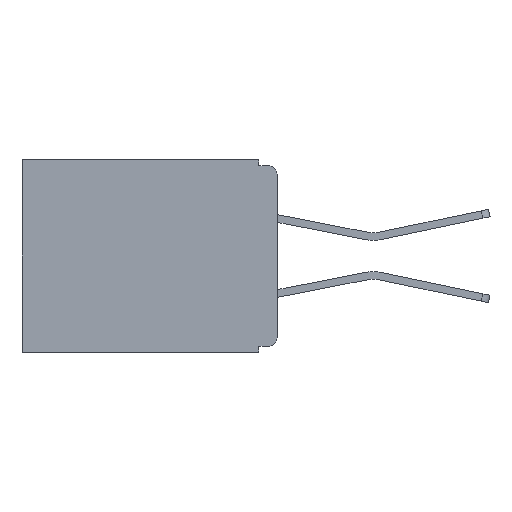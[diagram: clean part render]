
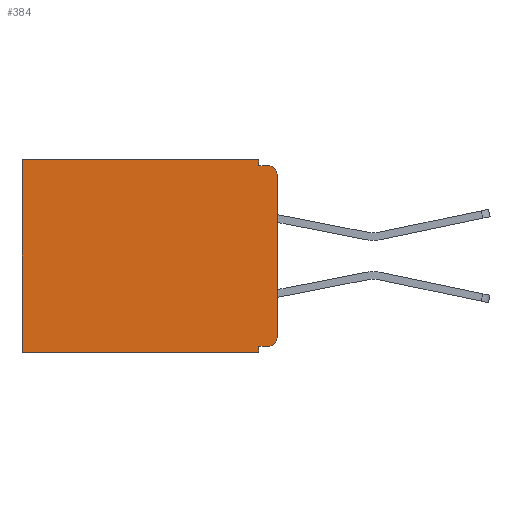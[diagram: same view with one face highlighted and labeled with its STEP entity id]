
A CAD part, left-side view. The second image highlights one B-rep face of the part: STEP entity #384.
In plain terms, the highlighted planar face has unit normal (-1, 0, 0).
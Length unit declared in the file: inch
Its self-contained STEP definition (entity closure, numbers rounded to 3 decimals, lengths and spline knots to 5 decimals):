
#215 = ORIENTED_EDGE ( 'NONE', *, *, #18705, .T. ) ;
#384 = ADVANCED_FACE ( 'NONE', ( #16890 ), #3548, .F. ) ;
#388 = DIRECTION ( 'NONE',  ( 0., -1., 0. ) ) ;
#589 = VERTEX_POINT ( 'NONE', #16058 ) ;
#838 = VECTOR ( 'NONE', #5993, 39.37008 ) ;
#1150 = VERTEX_POINT ( 'NONE', #18257 ) ;
#1849 = ORIENTED_EDGE ( 'NONE', *, *, #3924, .F. ) ;
#2258 = VERTEX_POINT ( 'NONE', #3129 ) ;
#2694 = CIRCLE ( 'NONE', #17497, 0.015 ) ;
#2860 = CARTESIAN_POINT ( 'NONE',  ( 0.3, 0., -0.33 ) ) ;
#3067 = DIRECTION ( 'NONE',  ( 0., 0., -1. ) ) ;
#3129 = CARTESIAN_POINT ( 'NONE',  ( 0.3, 0.437, -0.33 ) ) ;
#3267 = DIRECTION ( 'NONE',  ( 0., 0., -1. ) ) ;
#3391 = EDGE_CURVE ( 'NONE', #7942, #2258, #20672, .T. ) ;
#3458 = AXIS2_PLACEMENT_3D ( 'NONE', #2860, #11331, #7183 ) ;
#3548 = PLANE ( 'NONE',  #3458 ) ;
#3601 = DIRECTION ( 'NONE',  ( -1., 0., 0. ) ) ;
#3924 = EDGE_CURVE ( 'NONE', #12641, #8187, #18591, .T. ) ;
#4865 = VERTEX_POINT ( 'NONE', #8787 ) ;
#4877 = DIRECTION ( 'NONE',  ( -1., 0., 0. ) ) ;
#5636 = VECTOR ( 'NONE', #9084, 39.37008 ) ;
#5761 = CARTESIAN_POINT ( 'NONE',  ( 0.3, 0.031, -0.33 ) ) ;
#5874 = EDGE_CURVE ( 'NONE', #18102, #14571, #18915, .T. ) ;
#5951 = VECTOR ( 'NONE', #10264, 39.37008 ) ;
#5993 = DIRECTION ( 'NONE',  ( 0., 0., -1. ) ) ;
#6126 = EDGE_CURVE ( 'NONE', #15935, #2258, #9848, .T. ) ;
#6602 = CARTESIAN_POINT ( 'NONE',  ( 0.3, 0.437, 0. ) ) ;
#7183 = DIRECTION ( 'NONE',  ( 0., 0., -1. ) ) ;
#7385 = CARTESIAN_POINT ( 'NONE',  ( 0.3, 0., -0.01 ) ) ;
#7942 = VERTEX_POINT ( 'NONE', #5761 ) ;
#8187 = VERTEX_POINT ( 'NONE', #16365 ) ;
#8632 = CIRCLE ( 'NONE', #21584, 0.015 ) ;
#8787 = CARTESIAN_POINT ( 'NONE',  ( 0.3, 0.031, -0.32 ) ) ;
#9084 = DIRECTION ( 'NONE',  ( 0., 0., -1. ) ) ;
#9246 = CARTESIAN_POINT ( 'NONE',  ( 0.3, 0.031, -0.01 ) ) ;
#9286 = ORIENTED_EDGE ( 'NONE', *, *, #10385, .F. ) ;
#9453 = CARTESIAN_POINT ( 'NONE',  ( 0.3, 0., -0.33 ) ) ;
#9590 = CARTESIAN_POINT ( 'NONE',  ( 0.3, 0., -0.32 ) ) ;
#9814 = VECTOR ( 'NONE', #388, 39.37008 ) ;
#9848 = LINE ( 'NONE', #10572, #838 ) ;
#9910 = EDGE_CURVE ( 'NONE', #589, #4865, #11304, .T. ) ;
#10203 = VECTOR ( 'NONE', #3067, 39.37008 ) ;
#10264 = DIRECTION ( 'NONE',  ( 0., 1., 0. ) ) ;
#10385 = EDGE_CURVE ( 'NONE', #1150, #12641, #10756, .T. ) ;
#10405 = ORIENTED_EDGE ( 'NONE', *, *, #21154, .F. ) ;
#10423 = LINE ( 'NONE', #16744, #5951 ) ;
#10572 = CARTESIAN_POINT ( 'NONE',  ( 0.3, 0.437, -0.33 ) ) ;
#10644 = VECTOR ( 'NONE', #3267, 39.37008 ) ;
#10756 = LINE ( 'NONE', #14755, #10203 ) ;
#10833 = ORIENTED_EDGE ( 'NONE', *, *, #6126, .T. ) ;
#11304 = LINE ( 'NONE', #9590, #20042 ) ;
#11331 = DIRECTION ( 'NONE',  ( 1., 0., 0. ) ) ;
#11682 = DIRECTION ( 'NONE',  ( 0., 1., 0. ) ) ;
#11952 = VECTOR ( 'NONE', #11682, 39.37008 ) ;
#12263 = ORIENTED_EDGE ( 'NONE', *, *, #21543, .T. ) ;
#12641 = VERTEX_POINT ( 'NONE', #9246 ) ;
#13071 = ORIENTED_EDGE ( 'NONE', *, *, #16699, .T. ) ;
#13619 = CARTESIAN_POINT ( 'NONE',  ( 0.3, 0.015, -0.305 ) ) ;
#13903 = ORIENTED_EDGE ( 'NONE', *, *, #3391, .F. ) ;
#14571 = VERTEX_POINT ( 'NONE', #16184 ) ;
#14755 = CARTESIAN_POINT ( 'NONE',  ( 0.3, 0.031, 0. ) ) ;
#14851 = CARTESIAN_POINT ( 'NONE',  ( 0.3, 0.015, -0.025 ) ) ;
#15286 = DIRECTION ( 'NONE',  ( 0., 0., -1. ) ) ;
#15692 = CARTESIAN_POINT ( 'NONE',  ( 0.3, 0., -0.025 ) ) ;
#15935 = VERTEX_POINT ( 'NONE', #6602 ) ;
#16058 = CARTESIAN_POINT ( 'NONE',  ( 0.3, 0.015, -0.32 ) ) ;
#16184 = CARTESIAN_POINT ( 'NONE',  ( 0.3, 0., -0.305 ) ) ;
#16365 = CARTESIAN_POINT ( 'NONE',  ( 0.3, 0.015, -0.01 ) ) ;
#16494 = DIRECTION ( 'NONE',  ( 0., 0., -1. ) ) ;
#16699 = EDGE_CURVE ( 'NONE', #1150, #15935, #10423, .T. ) ;
#16744 = CARTESIAN_POINT ( 'NONE',  ( 0.3, 0., 0. ) ) ;
#16890 = FACE_OUTER_BOUND ( 'NONE', #17245, .T. ) ;
#17245 = EDGE_LOOP ( 'NONE', ( #21298, #215, #1849, #9286, #13071, #10833, #13903, #10405, #18028, #12263 ) ) ;
#17497 = AXIS2_PLACEMENT_3D ( 'NONE', #13619, #3601, #15286 ) ;
#18028 = ORIENTED_EDGE ( 'NONE', *, *, #9910, .F. ) ;
#18102 = VERTEX_POINT ( 'NONE', #15692 ) ;
#18257 = CARTESIAN_POINT ( 'NONE',  ( 0.3, 0.031, 0. ) ) ;
#18301 = CARTESIAN_POINT ( 'NONE',  ( 0.3, 0.031, -0.33 ) ) ;
#18591 = LINE ( 'NONE', #7385, #9814 ) ;
#18705 = EDGE_CURVE ( 'NONE', #18102, #8187, #8632, .T. ) ;
#18915 = LINE ( 'NONE', #20629, #5636 ) ;
#19428 = LINE ( 'NONE', #18301, #10644 ) ;
#20042 = VECTOR ( 'NONE', #21135, 39.37008 ) ;
#20629 = CARTESIAN_POINT ( 'NONE',  ( 0.3, 0., -0.33 ) ) ;
#20672 = LINE ( 'NONE', #9453, #11952 ) ;
#21135 = DIRECTION ( 'NONE',  ( 0., 1., 0. ) ) ;
#21154 = EDGE_CURVE ( 'NONE', #4865, #7942, #19428, .T. ) ;
#21298 = ORIENTED_EDGE ( 'NONE', *, *, #5874, .F. ) ;
#21543 = EDGE_CURVE ( 'NONE', #589, #14571, #2694, .T. ) ;
#21584 = AXIS2_PLACEMENT_3D ( 'NONE', #14851, #4877, #16494 ) ;
